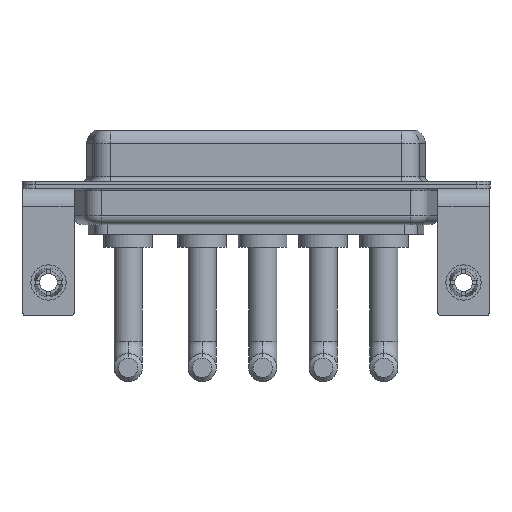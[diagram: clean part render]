
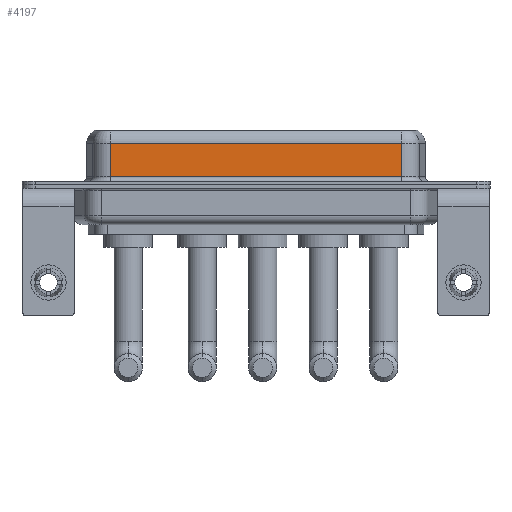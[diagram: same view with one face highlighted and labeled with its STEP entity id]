
A CAD part, front view. The second image highlights one B-rep face of the part: STEP entity #4197.
In plain terms, the highlighted planar face has unit normal (0, -1, 0).
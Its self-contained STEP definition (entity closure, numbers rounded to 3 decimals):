
#87 = AXIS2_PLACEMENT_3D ( 'NONE', #12119, #9702, #6154 ) ;
#759 = CARTESIAN_POINT ( 'NONE',  ( 40.037, -3.95, 4.65 ) ) ;
#1538 = EDGE_LOOP ( 'NONE', ( #2061, #3486, #8234, #9155 ) ) ;
#2061 = ORIENTED_EDGE ( 'NONE', *, *, #6566, .F. ) ;
#2530 = CARTESIAN_POINT ( 'NONE',  ( 7.013, -3.95, 6.4 ) ) ;
#3260 = VERTEX_POINT ( 'NONE', #12085 ) ;
#3486 = ORIENTED_EDGE ( 'NONE', *, *, #11663, .T. ) ;
#4197 = ADVANCED_FACE ( 'NONE', ( #14658 ), #5098, .F. ) ;
#4828 = DIRECTION ( 'NONE',  ( 0., 0., -1. ) ) ;
#5098 = PLANE ( 'NONE',  #87 ) ;
#6034 = CARTESIAN_POINT ( 'NONE',  ( 40.037, -3.95, 4.65 ) ) ;
#6049 = LINE ( 'NONE', #13316, #13517 ) ;
#6154 = DIRECTION ( 'NONE',  ( 0., 0., 1. ) ) ;
#6271 = DIRECTION ( 'NONE',  ( -1., 0., 0. ) ) ;
#6441 = CARTESIAN_POINT ( 'NONE',  ( 40.037, -3.95, 0.9 ) ) ;
#6566 = EDGE_CURVE ( 'NONE', #10267, #9793, #6049, .T. ) ;
#6809 = LINE ( 'NONE', #14068, #14786 ) ;
#7498 = LINE ( 'NONE', #6034, #13059 ) ;
#8175 = VECTOR ( 'NONE', #4828, 1000. ) ;
#8234 = ORIENTED_EDGE ( 'NONE', *, *, #13259, .T. ) ;
#9155 = ORIENTED_EDGE ( 'NONE', *, *, #11416, .T. ) ;
#9702 = DIRECTION ( 'NONE',  ( 0., 1., 0. ) ) ;
#9793 = VERTEX_POINT ( 'NONE', #6441 ) ;
#10267 = VERTEX_POINT ( 'NONE', #759 ) ;
#11302 = VERTEX_POINT ( 'NONE', #14912 ) ;
#11416 = EDGE_CURVE ( 'NONE', #11302, #9793, #6809, .T. ) ;
#11663 = EDGE_CURVE ( 'NONE', #10267, #3260, #7498, .T. ) ;
#12085 = CARTESIAN_POINT ( 'NONE',  ( 7.013, -3.95, 4.65 ) ) ;
#12119 = CARTESIAN_POINT ( 'NONE',  ( 40.037, -3.95, 6.4 ) ) ;
#12836 = DIRECTION ( 'NONE',  ( 1., 0., 0. ) ) ;
#12987 = LINE ( 'NONE', #2530, #8175 ) ;
#13059 = VECTOR ( 'NONE', #6271, 1000. ) ;
#13087 = DIRECTION ( 'NONE',  ( 0., 0., -1. ) ) ;
#13259 = EDGE_CURVE ( 'NONE', #3260, #11302, #12987, .T. ) ;
#13316 = CARTESIAN_POINT ( 'NONE',  ( 40.037, -3.95, 6.4 ) ) ;
#13517 = VECTOR ( 'NONE', #13087, 1000. ) ;
#14068 = CARTESIAN_POINT ( 'NONE',  ( 40.037, -3.95, 0.9 ) ) ;
#14658 = FACE_OUTER_BOUND ( 'NONE', #1538, .T. ) ;
#14786 = VECTOR ( 'NONE', #12836, 1000. ) ;
#14912 = CARTESIAN_POINT ( 'NONE',  ( 7.013, -3.95, 0.9 ) ) ;
